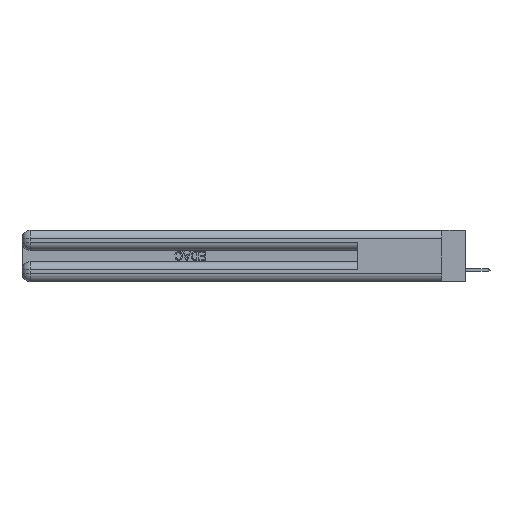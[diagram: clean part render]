
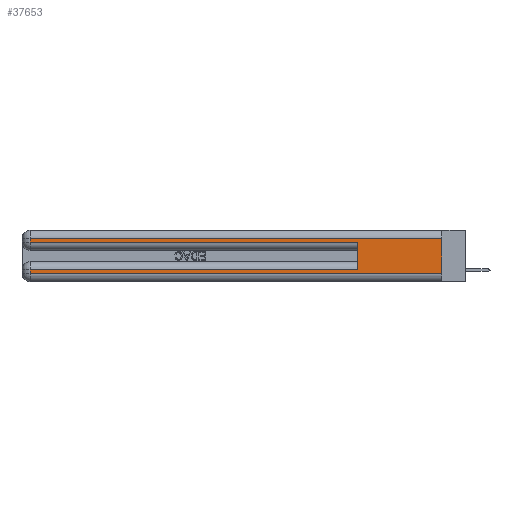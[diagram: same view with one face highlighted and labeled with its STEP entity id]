
A CAD part, left-side view. The second image highlights one B-rep face of the part: STEP entity #37653.
In plain terms, the highlighted planar face has unit normal (-1, 0, 0).
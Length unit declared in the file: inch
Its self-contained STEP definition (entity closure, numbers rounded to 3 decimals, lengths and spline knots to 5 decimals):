
#259 = CARTESIAN_POINT ( 'NONE',  ( 0., 0.6, 0.085 ) ) ;
#409 = VECTOR ( 'NONE', #10553, 39.37008 ) ;
#509 = CARTESIAN_POINT ( 'NONE',  ( 0., 2.94, 0.37 ) ) ;
#1249 = ORIENTED_EDGE ( 'NONE', *, *, #14879, .T. ) ;
#2335 = EDGE_CURVE ( 'NONE', #41970, #30927, #9375, .T. ) ;
#4241 = CARTESIAN_POINT ( 'NONE',  ( 0., 0., 0.285 ) ) ;
#5354 = VECTOR ( 'NONE', #37289, 39.37008 ) ;
#5503 = EDGE_LOOP ( 'NONE', ( #41297, #16325, #37696, #42830, #20244, #1249, #14023, #22595 ) ) ;
#7950 = LINE ( 'NONE', #4241, #36666 ) ;
#8020 = CARTESIAN_POINT ( 'NONE',  ( 0., 0., 0.06 ) ) ;
#8166 = DIRECTION ( 'NONE',  ( 0., -1., 0. ) ) ;
#9375 = LINE ( 'NONE', #30522, #409 ) ;
#9850 = CARTESIAN_POINT ( 'NONE',  ( 0., 0.6, 0.285 ) ) ;
#10482 = LINE ( 'NONE', #16395, #13135 ) ;
#10553 = DIRECTION ( 'NONE',  ( 0., 0., 1. ) ) ;
#11123 = FACE_OUTER_BOUND ( 'NONE', #5503, .T. ) ;
#12082 = PLANE ( 'NONE',  #17808 ) ;
#12115 = CARTESIAN_POINT ( 'NONE',  ( 0., 0., 0.31 ) ) ;
#12141 = CARTESIAN_POINT ( 'NONE',  ( 0., 0., 0.37 ) ) ;
#12829 = VERTEX_POINT ( 'NONE', #21436 ) ;
#13135 = VECTOR ( 'NONE', #33040, 39.37008 ) ;
#13269 = CARTESIAN_POINT ( 'NONE',  ( 0., 2.94, 0.085 ) ) ;
#14023 = ORIENTED_EDGE ( 'NONE', *, *, #38710, .T. ) ;
#14879 = EDGE_CURVE ( 'NONE', #41970, #34205, #40762, .T. ) ;
#15082 = VERTEX_POINT ( 'NONE', #37742 ) ;
#16325 = ORIENTED_EDGE ( 'NONE', *, *, #40728, .T. ) ;
#16395 = CARTESIAN_POINT ( 'NONE',  ( 0., 2.94, 0.37 ) ) ;
#16471 = CARTESIAN_POINT ( 'NONE',  ( 0., 0., 0.085 ) ) ;
#17395 = CARTESIAN_POINT ( 'NONE',  ( 0., 2.94, 0.285 ) ) ;
#17808 = AXIS2_PLACEMENT_3D ( 'NONE', #35694, #18762, #42091 ) ;
#18762 = DIRECTION ( 'NONE',  ( 1., 0., 0. ) ) ;
#19933 = DIRECTION ( 'NONE',  ( 0., 1., 0. ) ) ;
#20244 = ORIENTED_EDGE ( 'NONE', *, *, #2335, .F. ) ;
#20561 = DIRECTION ( 'NONE',  ( 0., -1., 0. ) ) ;
#21436 = CARTESIAN_POINT ( 'NONE',  ( 0., 2.94, 0.06 ) ) ;
#21923 = VECTOR ( 'NONE', #30169, 39.37008 ) ;
#22168 = CARTESIAN_POINT ( 'NONE',  ( 0., 2.94, 0.31 ) ) ;
#22237 = EDGE_CURVE ( 'NONE', #12829, #15082, #29226, .T. ) ;
#22564 = EDGE_CURVE ( 'NONE', #29495, #15082, #33362, .T. ) ;
#22595 = ORIENTED_EDGE ( 'NONE', *, *, #22237, .T. ) ;
#23237 = EDGE_CURVE ( 'NONE', #31628, #30927, #7950, .T. ) ;
#24430 = VECTOR ( 'NONE', #32733, 39.37008 ) ;
#24434 = LINE ( 'NONE', #40206, #38557 ) ;
#29226 = LINE ( 'NONE', #8020, #40693 ) ;
#29495 = VERTEX_POINT ( 'NONE', #12115 ) ;
#30169 = DIRECTION ( 'NONE',  ( 0., 1., 0. ) ) ;
#30522 = CARTESIAN_POINT ( 'NONE',  ( 0., 0.6, 0.145 ) ) ;
#30927 = VERTEX_POINT ( 'NONE', #9850 ) ;
#31433 = VERTEX_POINT ( 'NONE', #22168 ) ;
#31628 = VERTEX_POINT ( 'NONE', #17395 ) ;
#32733 = DIRECTION ( 'NONE',  ( 0., 0., -1. ) ) ;
#33040 = DIRECTION ( 'NONE',  ( 0., 0., -1. ) ) ;
#33362 = LINE ( 'NONE', #12141, #24430 ) ;
#34205 = VERTEX_POINT ( 'NONE', #13269 ) ;
#35694 = CARTESIAN_POINT ( 'NONE',  ( 0., 0., 0.37 ) ) ;
#36666 = VECTOR ( 'NONE', #20561, 39.37008 ) ;
#37289 = DIRECTION ( 'NONE',  ( 0., 0., -1. ) ) ;
#37653 = ADVANCED_FACE ( 'NONE', ( #11123 ), #12082, .F. ) ;
#37696 = ORIENTED_EDGE ( 'NONE', *, *, #37784, .T. ) ;
#37742 = CARTESIAN_POINT ( 'NONE',  ( 0., 0., 0.06 ) ) ;
#37784 = EDGE_CURVE ( 'NONE', #31433, #31628, #42921, .T. ) ;
#38557 = VECTOR ( 'NONE', #19933, 39.37008 ) ;
#38710 = EDGE_CURVE ( 'NONE', #34205, #12829, #10482, .T. ) ;
#40206 = CARTESIAN_POINT ( 'NONE',  ( 0., 0., 0.31 ) ) ;
#40693 = VECTOR ( 'NONE', #8166, 39.37008 ) ;
#40728 = EDGE_CURVE ( 'NONE', #29495, #31433, #24434, .T. ) ;
#40762 = LINE ( 'NONE', #16471, #21923 ) ;
#41297 = ORIENTED_EDGE ( 'NONE', *, *, #22564, .F. ) ;
#41970 = VERTEX_POINT ( 'NONE', #259 ) ;
#42091 = DIRECTION ( 'NONE',  ( 0., 0., -1. ) ) ;
#42830 = ORIENTED_EDGE ( 'NONE', *, *, #23237, .T. ) ;
#42921 = LINE ( 'NONE', #509, #5354 ) ;
